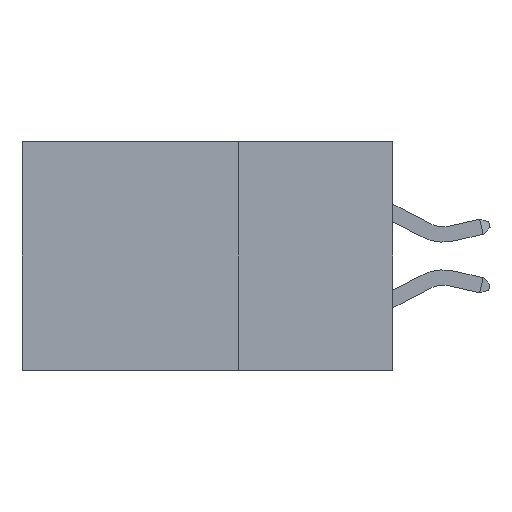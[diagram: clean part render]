
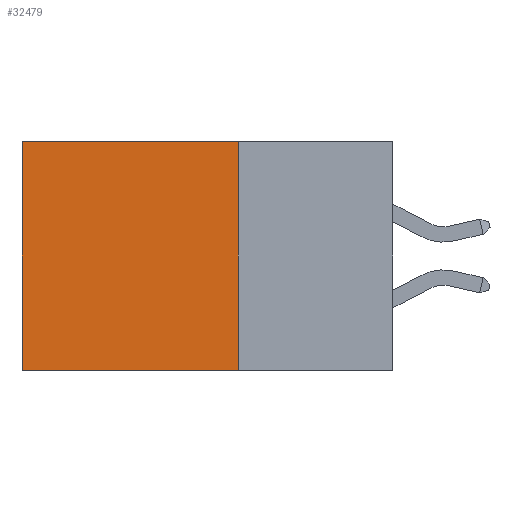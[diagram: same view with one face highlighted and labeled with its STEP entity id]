
A CAD part, left-side view. The second image highlights one B-rep face of the part: STEP entity #32479.
In plain terms, the highlighted planar face has unit normal (-1, 0, 0).
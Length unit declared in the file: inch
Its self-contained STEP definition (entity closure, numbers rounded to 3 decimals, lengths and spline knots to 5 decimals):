
#68 = LINE ( 'NONE', #10419, #26132 ) ;
#2065 = FACE_OUTER_BOUND ( 'NONE', #16280, .T. ) ;
#2273 = ORIENTED_EDGE ( 'NONE', *, *, #5766, .F. ) ;
#2740 = LINE ( 'NONE', #31284, #32519 ) ;
#3253 = ORIENTED_EDGE ( 'NONE', *, *, #21576, .T. ) ;
#4225 = PLANE ( 'NONE',  #4922 ) ;
#4277 = VERTEX_POINT ( 'NONE', #8775 ) ;
#4922 = AXIS2_PLACEMENT_3D ( 'NONE', #9068, #27271, #14592 ) ;
#4992 = ORIENTED_EDGE ( 'NONE', *, *, #14998, .F. ) ;
#5285 = DIRECTION ( 'NONE',  ( 0., 0., -1. ) ) ;
#5725 = DIRECTION ( 'NONE',  ( 0., 1., 0. ) ) ;
#5766 = EDGE_CURVE ( 'NONE', #24849, #8741, #2740, .T. ) ;
#8741 = VERTEX_POINT ( 'NONE', #32147 ) ;
#8775 = CARTESIAN_POINT ( 'NONE',  ( 0.2875, 0.6, 0. ) ) ;
#9068 = CARTESIAN_POINT ( 'NONE',  ( 0.2875, 0.25, 0. ) ) ;
#9672 = VECTOR ( 'NONE', #5285, 39.37008 ) ;
#10326 = EDGE_CURVE ( 'NONE', #4277, #29820, #28168, .T. ) ;
#10419 = CARTESIAN_POINT ( 'NONE',  ( 0.2875, 0.25, -0.37 ) ) ;
#12013 = CARTESIAN_POINT ( 'NONE',  ( 0.2875, 0.6, -0.37 ) ) ;
#14592 = DIRECTION ( 'NONE',  ( 0., 0., -1. ) ) ;
#14808 = ORIENTED_EDGE ( 'NONE', *, *, #10326, .T. ) ;
#14998 = EDGE_CURVE ( 'NONE', #8741, #29820, #68, .T. ) ;
#15630 = CARTESIAN_POINT ( 'NONE',  ( 0.2875, 0.6, 0. ) ) ;
#16280 = EDGE_LOOP ( 'NONE', ( #14808, #4992, #2273, #3253 ) ) ;
#21576 = EDGE_CURVE ( 'NONE', #24849, #4277, #29346, .T. ) ;
#21829 = DIRECTION ( 'NONE',  ( 0., 1., 0. ) ) ;
#24340 = CARTESIAN_POINT ( 'NONE',  ( 0.2875, 0.25, 0. ) ) ;
#24849 = VERTEX_POINT ( 'NONE', #29703 ) ;
#25944 = DIRECTION ( 'NONE',  ( 0., 0., -1. ) ) ;
#26132 = VECTOR ( 'NONE', #5725, 39.37008 ) ;
#27271 = DIRECTION ( 'NONE',  ( 1., 0., 0. ) ) ;
#27424 = VECTOR ( 'NONE', #21829, 39.37008 ) ;
#28168 = LINE ( 'NONE', #15630, #9672 ) ;
#29346 = LINE ( 'NONE', #24340, #27424 ) ;
#29703 = CARTESIAN_POINT ( 'NONE',  ( 0.2875, 0.25, 0. ) ) ;
#29820 = VERTEX_POINT ( 'NONE', #12013 ) ;
#31284 = CARTESIAN_POINT ( 'NONE',  ( 0.2875, 0.25, 0. ) ) ;
#32147 = CARTESIAN_POINT ( 'NONE',  ( 0.2875, 0.25, -0.37 ) ) ;
#32479 = ADVANCED_FACE ( 'NONE', ( #2065 ), #4225, .F. ) ;
#32519 = VECTOR ( 'NONE', #25944, 39.37008 ) ;
